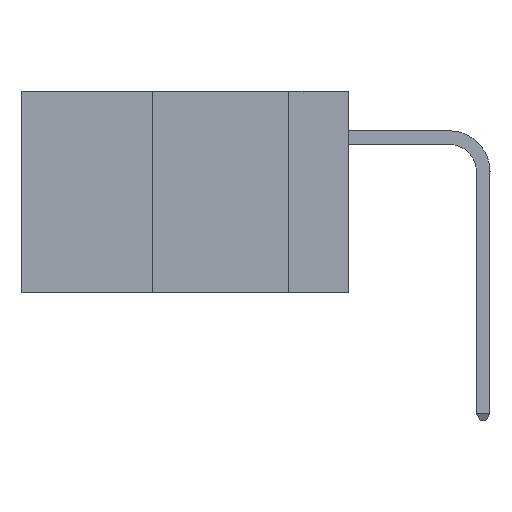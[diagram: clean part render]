
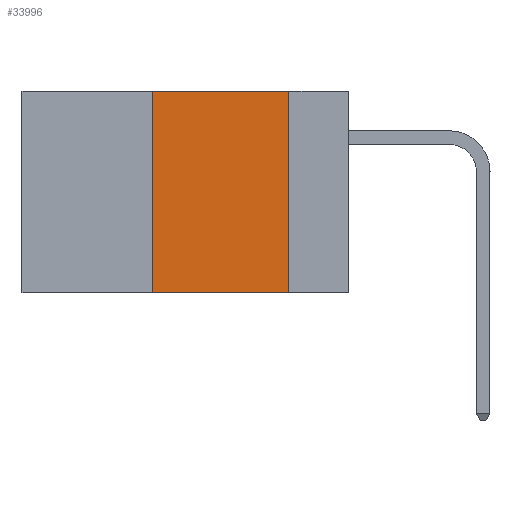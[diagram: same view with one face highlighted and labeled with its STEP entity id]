
A CAD part, left-side view. The second image highlights one B-rep face of the part: STEP entity #33996.
In plain terms, the highlighted planar face has unit normal (-1, 0, 0).
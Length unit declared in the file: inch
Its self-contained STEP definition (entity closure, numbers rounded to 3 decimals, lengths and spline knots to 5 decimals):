
#220 = ORIENTED_EDGE ( 'NONE', *, *, #11791, .T. ) ;
#888 = DIRECTION ( 'NONE',  ( 0., 0., -1. ) ) ;
#1045 = LINE ( 'NONE', #1486, #15055 ) ;
#1486 = CARTESIAN_POINT ( 'NONE',  ( 0., 0.36, 0. ) ) ;
#1710 = EDGE_LOOP ( 'NONE', ( #33474, #12448, #30798, #220 ) ) ;
#4022 = VERTEX_POINT ( 'NONE', #27280 ) ;
#4314 = DIRECTION ( 'NONE',  ( 0., 0., 1. ) ) ;
#5332 = DIRECTION ( 'NONE',  ( 0., -1., 0. ) ) ;
#9751 = PLANE ( 'NONE',  #33693 ) ;
#10134 = DIRECTION ( 'NONE',  ( 0., -1., 0. ) ) ;
#10326 = LINE ( 'NONE', #14818, #15969 ) ;
#10697 = VECTOR ( 'NONE', #10134, 39.37008 ) ;
#11528 = CARTESIAN_POINT ( 'NONE',  ( 0., 0.11, -0.37 ) ) ;
#11791 = EDGE_CURVE ( 'NONE', #4022, #20505, #25471, .T. ) ;
#12448 = ORIENTED_EDGE ( 'NONE', *, *, #24411, .F. ) ;
#14818 = CARTESIAN_POINT ( 'NONE',  ( 0., 0.11, 0. ) ) ;
#15055 = VECTOR ( 'NONE', #4314, 39.37008 ) ;
#15341 = CARTESIAN_POINT ( 'NONE',  ( 0., 0.6, 0. ) ) ;
#15616 = CARTESIAN_POINT ( 'NONE',  ( 0., 0.6, -0.37 ) ) ;
#15969 = VECTOR ( 'NONE', #888, 39.37008 ) ;
#17241 = VERTEX_POINT ( 'NONE', #35051 ) ;
#17423 = FACE_OUTER_BOUND ( 'NONE', #1710, .T. ) ;
#18141 = DIRECTION ( 'NONE',  ( 0., 0., -1. ) ) ;
#19252 = EDGE_CURVE ( 'NONE', #4022, #17241, #1045, .T. ) ;
#19783 = CARTESIAN_POINT ( 'NONE',  ( 0., 0.11, 0. ) ) ;
#20094 = LINE ( 'NONE', #22039, #34898 ) ;
#20505 = VERTEX_POINT ( 'NONE', #11528 ) ;
#22039 = CARTESIAN_POINT ( 'NONE',  ( 0., 0.6, 0. ) ) ;
#24411 = EDGE_CURVE ( 'NONE', #17241, #27195, #20094, .T. ) ;
#25471 = LINE ( 'NONE', #15616, #10697 ) ;
#27195 = VERTEX_POINT ( 'NONE', #19783 ) ;
#27280 = CARTESIAN_POINT ( 'NONE',  ( 0., 0.36, -0.37 ) ) ;
#28576 = EDGE_CURVE ( 'NONE', #27195, #20505, #10326, .T. ) ;
#30798 = ORIENTED_EDGE ( 'NONE', *, *, #19252, .F. ) ;
#33474 = ORIENTED_EDGE ( 'NONE', *, *, #28576, .F. ) ;
#33693 = AXIS2_PLACEMENT_3D ( 'NONE', #15341, #34816, #18141 ) ;
#33996 = ADVANCED_FACE ( 'NONE', ( #17423 ), #9751, .F. ) ;
#34816 = DIRECTION ( 'NONE',  ( 1., 0., 0. ) ) ;
#34898 = VECTOR ( 'NONE', #5332, 39.37008 ) ;
#35051 = CARTESIAN_POINT ( 'NONE',  ( 0., 0.36, 0. ) ) ;
